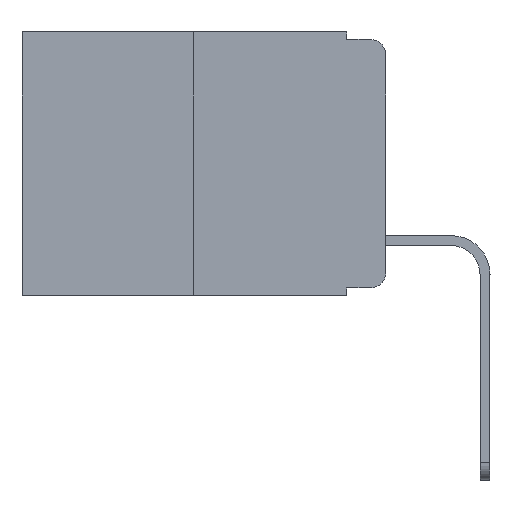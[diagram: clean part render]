
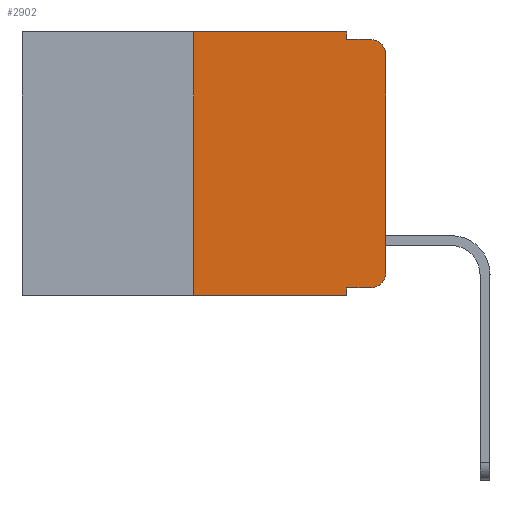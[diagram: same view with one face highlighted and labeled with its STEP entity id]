
A CAD part, left-side view. The second image highlights one B-rep face of the part: STEP entity #2902.
In plain terms, the highlighted planar face has unit normal (-1, 0, 0).
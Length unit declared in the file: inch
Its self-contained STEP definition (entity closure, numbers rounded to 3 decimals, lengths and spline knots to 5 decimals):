
#46 = VERTEX_POINT ( 'NONE', #17539 ) ;
#712 = CARTESIAN_POINT ( 'NONE',  ( 0., 0.473, 0. ) ) ;
#1061 = EDGE_CURVE ( 'NONE', #46, #12412, #15481, .T. ) ;
#1525 = CARTESIAN_POINT ( 'NONE',  ( 0., 0., -0.313 ) ) ;
#1797 = DIRECTION ( 'NONE',  ( 0., -1., 0. ) ) ;
#2794 = ORIENTED_EDGE ( 'NONE', *, *, #24169, .T. ) ;
#2869 = CARTESIAN_POINT ( 'NONE',  ( 0., 0.473, -0.343 ) ) ;
#2902 = ADVANCED_FACE ( 'NONE', ( #21581 ), #12724, .F. ) ;
#3240 = VECTOR ( 'NONE', #15172, 39.37008 ) ;
#3647 = VERTEX_POINT ( 'NONE', #8691 ) ;
#3769 = CARTESIAN_POINT ( 'NONE',  ( 0., 0.051, -0.333 ) ) ;
#3887 = DIRECTION ( 'NONE',  ( 0., 0., -1. ) ) ;
#3998 = CARTESIAN_POINT ( 'NONE',  ( 0., 0.051, -0.333 ) ) ;
#4136 = CARTESIAN_POINT ( 'NONE',  ( 0., 0.051, 0. ) ) ;
#4624 = ORIENTED_EDGE ( 'NONE', *, *, #10210, .F. ) ;
#4915 = EDGE_CURVE ( 'NONE', #14858, #3647, #9427, .T. ) ;
#5008 = ORIENTED_EDGE ( 'NONE', *, *, #16970, .F. ) ;
#5799 = DIRECTION ( 'NONE',  ( 0., 0., 1. ) ) ;
#5806 = EDGE_LOOP ( 'NONE', ( #2794, #19041, #13354, #5008, #21100, #8503, #18203, #4624, #8623, #23919 ) ) ;
#5833 = AXIS2_PLACEMENT_3D ( 'NONE', #24173, #18562, #23923 ) ;
#6051 = AXIS2_PLACEMENT_3D ( 'NONE', #22093, #8860, #22168 ) ;
#6437 = EDGE_CURVE ( 'NONE', #18527, #6723, #6441, .T. ) ;
#6441 = LINE ( 'NONE', #22398, #7305 ) ;
#6488 = VERTEX_POINT ( 'NONE', #22647 ) ;
#6723 = VERTEX_POINT ( 'NONE', #12826 ) ;
#7305 = VECTOR ( 'NONE', #1797, 39.37008 ) ;
#8503 = ORIENTED_EDGE ( 'NONE', *, *, #22176, .F. ) ;
#8623 = ORIENTED_EDGE ( 'NONE', *, *, #4915, .T. ) ;
#8691 = CARTESIAN_POINT ( 'NONE',  ( 0., 0.02, -0.333 ) ) ;
#8815 = EDGE_CURVE ( 'NONE', #19512, #15491, #19499, .T. ) ;
#8860 = DIRECTION ( 'NONE',  ( 1., 0., 0. ) ) ;
#9427 = LINE ( 'NONE', #3769, #3240 ) ;
#10210 = EDGE_CURVE ( 'NONE', #14858, #12412, #16471, .T. ) ;
#11342 = VECTOR ( 'NONE', #20778, 39.37008 ) ;
#11771 = VECTOR ( 'NONE', #12832, 39.37008 ) ;
#12091 = CIRCLE ( 'NONE', #5833, 0.02 ) ;
#12246 = VECTOR ( 'NONE', #20012, 39.37008 ) ;
#12412 = VERTEX_POINT ( 'NONE', #19733 ) ;
#12724 = PLANE ( 'NONE',  #6051 ) ;
#12826 = CARTESIAN_POINT ( 'NONE',  ( 0., 0.02, -0.01 ) ) ;
#12832 = DIRECTION ( 'NONE',  ( 0., 0., -1. ) ) ;
#13354 = ORIENTED_EDGE ( 'NONE', *, *, #6437, .F. ) ;
#13666 = DIRECTION ( 'NONE',  ( 0., -1., 0. ) ) ;
#14446 = CARTESIAN_POINT ( 'NONE',  ( 0., 0.051, -0.01 ) ) ;
#14858 = VERTEX_POINT ( 'NONE', #3998 ) ;
#15073 = CARTESIAN_POINT ( 'NONE',  ( 0., 0.25, 0. ) ) ;
#15126 = DIRECTION ( 'NONE',  ( -1., 0., 0. ) ) ;
#15172 = DIRECTION ( 'NONE',  ( 0., -1., 0. ) ) ;
#15481 = LINE ( 'NONE', #2869, #12246 ) ;
#15491 = VERTEX_POINT ( 'NONE', #4136 ) ;
#16314 = LINE ( 'NONE', #16786, #11342 ) ;
#16471 = LINE ( 'NONE', #24350, #11771 ) ;
#16786 = CARTESIAN_POINT ( 'NONE',  ( 0., 0.051, 0. ) ) ;
#16970 = EDGE_CURVE ( 'NONE', #15491, #18527, #16314, .T. ) ;
#17198 = CARTESIAN_POINT ( 'NONE',  ( 0., 0., 0. ) ) ;
#17539 = CARTESIAN_POINT ( 'NONE',  ( 0., 0.25, -0.343 ) ) ;
#17903 = AXIS2_PLACEMENT_3D ( 'NONE', #22604, #15126, #3887 ) ;
#18203 = ORIENTED_EDGE ( 'NONE', *, *, #1061, .T. ) ;
#18527 = VERTEX_POINT ( 'NONE', #14446 ) ;
#18562 = DIRECTION ( 'NONE',  ( -1., 0., 0. ) ) ;
#19041 = ORIENTED_EDGE ( 'NONE', *, *, #20079, .T. ) ;
#19337 = LINE ( 'NONE', #17198, #23453 ) ;
#19499 = LINE ( 'NONE', #712, #20086 ) ;
#19512 = VERTEX_POINT ( 'NONE', #15073 ) ;
#19733 = CARTESIAN_POINT ( 'NONE',  ( 0., 0.051, -0.343 ) ) ;
#19855 = DIRECTION ( 'NONE',  ( 0., 0., 1. ) ) ;
#20012 = DIRECTION ( 'NONE',  ( 0., -1., 0. ) ) ;
#20079 = EDGE_CURVE ( 'NONE', #6488, #6723, #12091, .T. ) ;
#20086 = VECTOR ( 'NONE', #13666, 39.37008 ) ;
#20109 = EDGE_CURVE ( 'NONE', #3647, #23281, #23264, .T. ) ;
#20778 = DIRECTION ( 'NONE',  ( 0., 0., -1. ) ) ;
#21100 = ORIENTED_EDGE ( 'NONE', *, *, #8815, .F. ) ;
#21506 = VECTOR ( 'NONE', #19855, 39.37008 ) ;
#21581 = FACE_OUTER_BOUND ( 'NONE', #5806, .T. ) ;
#21853 = LINE ( 'NONE', #23814, #21506 ) ;
#22093 = CARTESIAN_POINT ( 'NONE',  ( 0., 0.473, 0. ) ) ;
#22168 = DIRECTION ( 'NONE',  ( 0., 0., -1. ) ) ;
#22176 = EDGE_CURVE ( 'NONE', #46, #19512, #21853, .T. ) ;
#22398 = CARTESIAN_POINT ( 'NONE',  ( 0., 0.051, -0.01 ) ) ;
#22604 = CARTESIAN_POINT ( 'NONE',  ( 0., 0.02, -0.313 ) ) ;
#22647 = CARTESIAN_POINT ( 'NONE',  ( 0., 0., -0.03 ) ) ;
#23264 = CIRCLE ( 'NONE', #17903, 0.02 ) ;
#23281 = VERTEX_POINT ( 'NONE', #1525 ) ;
#23453 = VECTOR ( 'NONE', #5799, 39.37008 ) ;
#23814 = CARTESIAN_POINT ( 'NONE',  ( 0., 0.25, 0. ) ) ;
#23919 = ORIENTED_EDGE ( 'NONE', *, *, #20109, .T. ) ;
#23923 = DIRECTION ( 'NONE',  ( 0., 0., -1. ) ) ;
#24169 = EDGE_CURVE ( 'NONE', #23281, #6488, #19337, .T. ) ;
#24173 = CARTESIAN_POINT ( 'NONE',  ( 0., 0.02, -0.03 ) ) ;
#24350 = CARTESIAN_POINT ( 'NONE',  ( 0., 0.051, 0. ) ) ;
